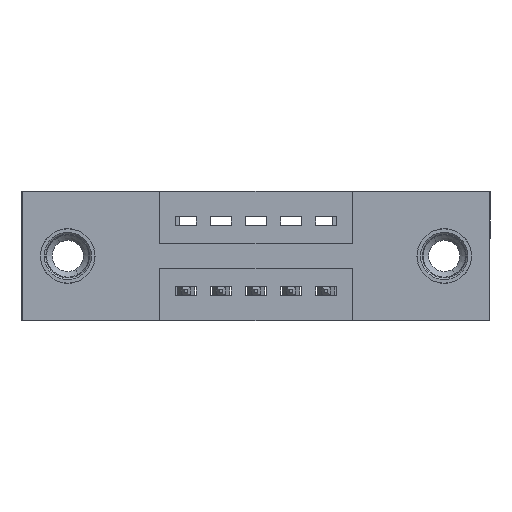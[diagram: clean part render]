
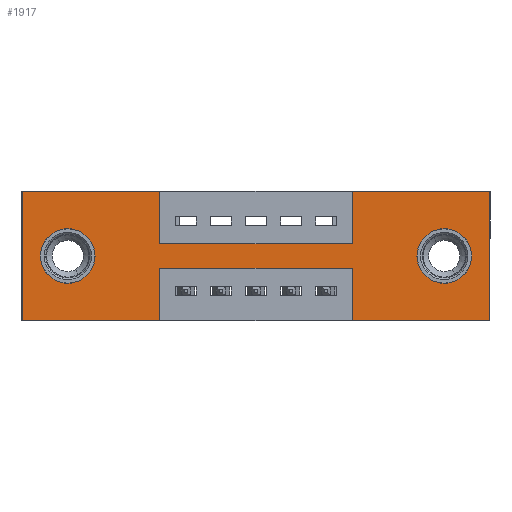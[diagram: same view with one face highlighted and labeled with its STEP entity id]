
A CAD part, front view. The second image highlights one B-rep face of the part: STEP entity #1917.
In plain terms, the highlighted planar face has unit normal (0, -1, 0).
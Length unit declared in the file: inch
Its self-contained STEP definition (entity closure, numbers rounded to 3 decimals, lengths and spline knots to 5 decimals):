
#8 = DIRECTION ( 'NONE',  ( 1., 0., 0. ) ) ;
#34 = VECTOR ( 'NONE', #6965, 39.37008 ) ;
#115 = ORIENTED_EDGE ( 'NONE', *, *, #10081, .F. ) ;
#174 = LINE ( 'NONE', #1706, #8883 ) ;
#302 = ORIENTED_EDGE ( 'NONE', *, *, #7019, .F. ) ;
#306 = EDGE_CURVE ( 'NONE', #7298, #4103, #4515, .T. ) ;
#331 = VECTOR ( 'NONE', #9907, 39.37008 ) ;
#370 = EDGE_CURVE ( 'NONE', #4103, #7298, #4176, .T. ) ;
#409 = VECTOR ( 'NONE', #10273, 39.37008 ) ;
#417 = CIRCLE ( 'NONE', #3430, 0.078 ) ;
#491 = VERTEX_POINT ( 'NONE', #8344 ) ;
#530 = LINE ( 'NONE', #8599, #409 ) ;
#687 = DIRECTION ( 'NONE',  ( 0., -1., 0. ) ) ;
#799 = EDGE_CURVE ( 'NONE', #8721, #8306, #1910, .T. ) ;
#830 = DIRECTION ( 'NONE',  ( 1., 0., 0. ) ) ;
#1049 = CARTESIAN_POINT ( 'NONE',  ( 0.9425, 0., -0.37 ) ) ;
#1233 = LINE ( 'NONE', #8231, #331 ) ;
#1315 = AXIS2_PLACEMENT_3D ( 'NONE', #6525, #687, #9845 ) ;
#1377 = AXIS2_PLACEMENT_3D ( 'NONE', #6260, #5385, #3659 ) ;
#1405 = ORIENTED_EDGE ( 'NONE', *, *, #10744, .F. ) ;
#1416 = ORIENTED_EDGE ( 'NONE', *, *, #9253, .F. ) ;
#1607 = LINE ( 'NONE', #1049, #34 ) ;
#1706 = CARTESIAN_POINT ( 'NONE',  ( 0.3925, 0., -0.22 ) ) ;
#1783 = VERTEX_POINT ( 'NONE', #10836 ) ;
#1833 = VERTEX_POINT ( 'NONE', #8478 ) ;
#1881 = VECTOR ( 'NONE', #8, 39.37008 ) ;
#1903 = EDGE_CURVE ( 'NONE', #8530, #9713, #6280, .T. ) ;
#1910 = CIRCLE ( 'NONE', #1377, 0.078 ) ;
#1917 = ADVANCED_FACE ( 'NONE', ( #2834, #9709, #7459 ), #4070, .T. ) ;
#2050 = CARTESIAN_POINT ( 'NONE',  ( 0.9425, 0., 0. ) ) ;
#2163 = DIRECTION ( 'NONE',  ( 0., 1., 0. ) ) ;
#2174 = ORIENTED_EDGE ( 'NONE', *, *, #4355, .F. ) ;
#2243 = EDGE_CURVE ( 'NONE', #8925, #8530, #1233, .T. ) ;
#2360 = VERTEX_POINT ( 'NONE', #4522 ) ;
#2440 = CARTESIAN_POINT ( 'NONE',  ( 0., 0., 0. ) ) ;
#2496 = VECTOR ( 'NONE', #8312, 39.37008 ) ;
#2498 = VECTOR ( 'NONE', #3879, 39.37008 ) ;
#2834 = FACE_BOUND ( 'NONE', #7780, .T. ) ;
#2903 = VECTOR ( 'NONE', #830, 39.37008 ) ;
#2948 = DIRECTION ( 'NONE',  ( 0., 0., 1. ) ) ;
#2978 = CARTESIAN_POINT ( 'NONE',  ( 0.13, 0., -0.263 ) ) ;
#2986 = CARTESIAN_POINT ( 'NONE',  ( 1.205, 0., -0.185 ) ) ;
#3059 = CARTESIAN_POINT ( 'NONE',  ( 0.9425, 0., 0. ) ) ;
#3130 = VERTEX_POINT ( 'NONE', #3653 ) ;
#3169 = ORIENTED_EDGE ( 'NONE', *, *, #3201, .F. ) ;
#3201 = EDGE_CURVE ( 'NONE', #6736, #3130, #174, .T. ) ;
#3430 = AXIS2_PLACEMENT_3D ( 'NONE', #2986, #3833, #5594 ) ;
#3524 = ORIENTED_EDGE ( 'NONE', *, *, #2243, .F. ) ;
#3653 = CARTESIAN_POINT ( 'NONE',  ( 0.3925, 0., -0.22 ) ) ;
#3659 = DIRECTION ( 'NONE',  ( 0., 0., -1. ) ) ;
#3706 = LINE ( 'NONE', #3059, #4633 ) ;
#3713 = CARTESIAN_POINT ( 'NONE',  ( 0.3925, 0., -0.15 ) ) ;
#3756 = LINE ( 'NONE', #5498, #2498 ) ;
#3833 = DIRECTION ( 'NONE',  ( 0., 1., 0. ) ) ;
#3846 = ORIENTED_EDGE ( 'NONE', *, *, #10043, .F. ) ;
#3879 = DIRECTION ( 'NONE',  ( 0., 0., -1. ) ) ;
#3890 = CARTESIAN_POINT ( 'NONE',  ( 0.3925, 0., 0. ) ) ;
#4070 = PLANE ( 'NONE',  #1315 ) ;
#4086 = ORIENTED_EDGE ( 'NONE', *, *, #1903, .F. ) ;
#4103 = VERTEX_POINT ( 'NONE', #2978 ) ;
#4176 = CIRCLE ( 'NONE', #9345, 0.078 ) ;
#4196 = VERTEX_POINT ( 'NONE', #6315 ) ;
#4213 = VECTOR ( 'NONE', #5297, 39.37008 ) ;
#4355 = EDGE_CURVE ( 'NONE', #8430, #4196, #10183, .T. ) ;
#4389 = ORIENTED_EDGE ( 'NONE', *, *, #6770, .F. ) ;
#4475 = VECTOR ( 'NONE', #8158, 39.37008 ) ;
#4515 = CIRCLE ( 'NONE', #10654, 0.078 ) ;
#4522 = CARTESIAN_POINT ( 'NONE',  ( 0., 0., -0.37 ) ) ;
#4633 = VECTOR ( 'NONE', #2948, 39.37008 ) ;
#4662 = CARTESIAN_POINT ( 'NONE',  ( 0.13, 0., -0.107 ) ) ;
#4726 = EDGE_CURVE ( 'NONE', #3130, #491, #3756, .T. ) ;
#5276 = CARTESIAN_POINT ( 'NONE',  ( 0.13, 0., -0.185 ) ) ;
#5287 = DIRECTION ( 'NONE',  ( 0., 0., -1. ) ) ;
#5297 = DIRECTION ( 'NONE',  ( 0., 0., 1. ) ) ;
#5370 = ORIENTED_EDGE ( 'NONE', *, *, #799, .T. ) ;
#5385 = DIRECTION ( 'NONE',  ( 0., 1., 0. ) ) ;
#5498 = CARTESIAN_POINT ( 'NONE',  ( 0.3925, 0., -0.37 ) ) ;
#5545 = CARTESIAN_POINT ( 'NONE',  ( 0.13, 0., -0.185 ) ) ;
#5594 = DIRECTION ( 'NONE',  ( 0., 0., -1. ) ) ;
#5964 = VERTEX_POINT ( 'NONE', #7545 ) ;
#6041 = CARTESIAN_POINT ( 'NONE',  ( 0., 0., 0. ) ) ;
#6148 = DIRECTION ( 'NONE',  ( -1., 0., 0. ) ) ;
#6158 = DIRECTION ( 'NONE',  ( 0., 0., 1. ) ) ;
#6260 = CARTESIAN_POINT ( 'NONE',  ( 1.205, 0., -0.185 ) ) ;
#6280 = LINE ( 'NONE', #7045, #6808 ) ;
#6315 = CARTESIAN_POINT ( 'NONE',  ( 1.335, 0., 0. ) ) ;
#6328 = CARTESIAN_POINT ( 'NONE',  ( 1.335, 0., 0. ) ) ;
#6525 = CARTESIAN_POINT ( 'NONE',  ( 0., 0., -0.37 ) ) ;
#6736 = VERTEX_POINT ( 'NONE', #8876 ) ;
#6770 = EDGE_CURVE ( 'NONE', #4196, #1833, #8958, .T. ) ;
#6808 = VECTOR ( 'NONE', #5287, 39.37008 ) ;
#6836 = CARTESIAN_POINT ( 'NONE',  ( 0., 0., 0. ) ) ;
#6958 = DIRECTION ( 'NONE',  ( 0., 1., 0. ) ) ;
#6965 = DIRECTION ( 'NONE',  ( 0., 0., 1. ) ) ;
#7019 = EDGE_CURVE ( 'NONE', #9713, #5964, #10348, .T. ) ;
#7045 = CARTESIAN_POINT ( 'NONE',  ( 0.3925, 0., 0. ) ) ;
#7143 = ORIENTED_EDGE ( 'NONE', *, *, #4726, .F. ) ;
#7258 = LINE ( 'NONE', #7444, #2496 ) ;
#7298 = VERTEX_POINT ( 'NONE', #4662 ) ;
#7402 = CARTESIAN_POINT ( 'NONE',  ( 1.205, 0., -0.263 ) ) ;
#7444 = CARTESIAN_POINT ( 'NONE',  ( 0., 0., -0.37 ) ) ;
#7459 = FACE_OUTER_BOUND ( 'NONE', #9108, .T. ) ;
#7545 = CARTESIAN_POINT ( 'NONE',  ( 0.9425, 0., -0.15 ) ) ;
#7779 = CARTESIAN_POINT ( 'NONE',  ( 1.205, 0., -0.107 ) ) ;
#7780 = EDGE_LOOP ( 'NONE', ( #9772, #5370 ) ) ;
#8097 = DIRECTION ( 'NONE',  ( 0., 0., 1. ) ) ;
#8158 = DIRECTION ( 'NONE',  ( 0., 0., -1. ) ) ;
#8231 = CARTESIAN_POINT ( 'NONE',  ( 0., 0., 0. ) ) ;
#8306 = VERTEX_POINT ( 'NONE', #7779 ) ;
#8312 = DIRECTION ( 'NONE',  ( -1., 0., 0. ) ) ;
#8344 = CARTESIAN_POINT ( 'NONE',  ( 0.3925, 0., -0.37 ) ) ;
#8414 = EDGE_CURVE ( 'NONE', #1783, #6736, #1607, .T. ) ;
#8430 = VERTEX_POINT ( 'NONE', #2050 ) ;
#8478 = CARTESIAN_POINT ( 'NONE',  ( 1.335, 0., -0.37 ) ) ;
#8530 = VERTEX_POINT ( 'NONE', #3890 ) ;
#8567 = ORIENTED_EDGE ( 'NONE', *, *, #370, .T. ) ;
#8582 = ORIENTED_EDGE ( 'NONE', *, *, #306, .T. ) ;
#8599 = CARTESIAN_POINT ( 'NONE',  ( 0., 0., -0.37 ) ) ;
#8721 = VERTEX_POINT ( 'NONE', #7402 ) ;
#8876 = CARTESIAN_POINT ( 'NONE',  ( 0.9425, 0., -0.22 ) ) ;
#8883 = VECTOR ( 'NONE', #6148, 39.37008 ) ;
#8925 = VERTEX_POINT ( 'NONE', #6041 ) ;
#8958 = LINE ( 'NONE', #6328, #4475 ) ;
#9108 = EDGE_LOOP ( 'NONE', ( #7143, #3169, #10678, #3846, #4389, #2174, #1416, #302, #4086, #3524, #1405, #115 ) ) ;
#9145 = EDGE_LOOP ( 'NONE', ( #8582, #8567 ) ) ;
#9253 = EDGE_CURVE ( 'NONE', #5964, #8430, #3706, .T. ) ;
#9322 = EDGE_CURVE ( 'NONE', #8306, #8721, #417, .T. ) ;
#9345 = AXIS2_PLACEMENT_3D ( 'NONE', #5276, #6958, #6158 ) ;
#9709 = FACE_BOUND ( 'NONE', #9145, .T. ) ;
#9713 = VERTEX_POINT ( 'NONE', #3713 ) ;
#9772 = ORIENTED_EDGE ( 'NONE', *, *, #9322, .T. ) ;
#9845 = DIRECTION ( 'NONE',  ( 0., 0., -1. ) ) ;
#9907 = DIRECTION ( 'NONE',  ( 1., 0., 0. ) ) ;
#10043 = EDGE_CURVE ( 'NONE', #1833, #1783, #7258, .T. ) ;
#10081 = EDGE_CURVE ( 'NONE', #491, #2360, #530, .T. ) ;
#10155 = CARTESIAN_POINT ( 'NONE',  ( 0.3925, 0., -0.15 ) ) ;
#10183 = LINE ( 'NONE', #2440, #2903 ) ;
#10273 = DIRECTION ( 'NONE',  ( -1., 0., 0. ) ) ;
#10348 = LINE ( 'NONE', #10155, #1881 ) ;
#10534 = LINE ( 'NONE', #6836, #4213 ) ;
#10654 = AXIS2_PLACEMENT_3D ( 'NONE', #5545, #2163, #8097 ) ;
#10678 = ORIENTED_EDGE ( 'NONE', *, *, #8414, .F. ) ;
#10744 = EDGE_CURVE ( 'NONE', #2360, #8925, #10534, .T. ) ;
#10836 = CARTESIAN_POINT ( 'NONE',  ( 0.9425, 0., -0.37 ) ) ;
